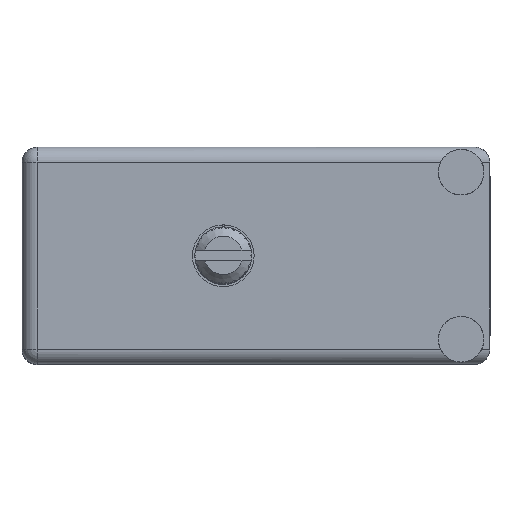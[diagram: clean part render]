
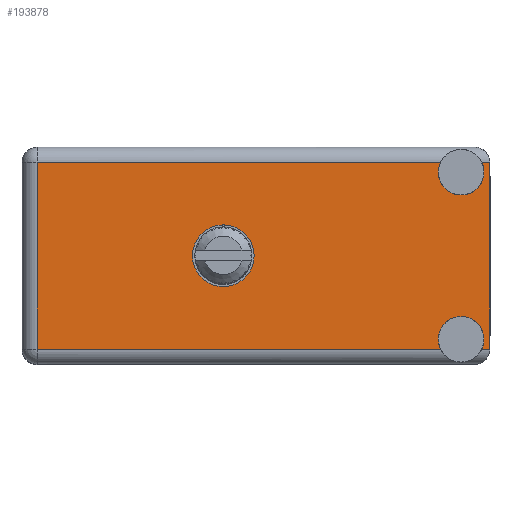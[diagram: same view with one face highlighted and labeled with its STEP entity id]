
A CAD part, top view. The second image highlights one B-rep face of the part: STEP entity #193878.
In plain terms, the highlighted face is planar.
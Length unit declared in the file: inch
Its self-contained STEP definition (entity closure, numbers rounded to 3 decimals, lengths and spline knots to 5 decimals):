
#703 = ORIENTED_EDGE ( 'NONE', *, *, #146968, .T. ) ;
#1648 = EDGE_CURVE ( 'NONE', #53307, #100496, #67177, .T. ) ;
#1703 = CIRCLE ( 'NONE', #99555, 0.1015 ) ;
#3553 = CARTESIAN_POINT ( 'NONE',  ( 0., 0.906, -0.665 ) ) ;
#8073 = DIRECTION ( 'NONE',  ( 0., 0., 1. ) ) ;
#11245 = CARTESIAN_POINT ( 'NONE',  ( 1.539, 0.906, -0.05 ) ) ;
#12957 = CARTESIAN_POINT ( 'NONE',  ( 0.6625, 0.906, -0.3575 ) ) ;
#14248 = CARTESIAN_POINT ( 'NONE',  ( 0.6625, 0.906, -0.459 ) ) ;
#14769 = ORIENTED_EDGE ( 'NONE', *, *, #183050, .F. ) ;
#20275 = VERTEX_POINT ( 'NONE', #14248 ) ;
#21609 = ORIENTED_EDGE ( 'NONE', *, *, #87381, .F. ) ;
#32112 = ORIENTED_EDGE ( 'NONE', *, *, #156382, .F. ) ;
#32458 = AXIS2_PLACEMENT_3D ( 'NONE', #95617, #155891, #96591 ) ;
#45005 = LINE ( 'NONE', #119097, #183199 ) ;
#48723 = CARTESIAN_POINT ( 'NONE',  ( 1.37741, 0.906, -0.05 ) ) ;
#49349 = CARTESIAN_POINT ( 'NONE',  ( 1.445, 0.906, -0.5575 ) ) ;
#52432 = CARTESIAN_POINT ( 'NONE',  ( 1.539, 0.906, -0.05 ) ) ;
#53307 = VERTEX_POINT ( 'NONE', #184322 ) ;
#53996 = DIRECTION ( 'NONE',  ( 0., 1., 0. ) ) ;
#55192 = CARTESIAN_POINT ( 'NONE',  ( 1.445, 0.906, -0.0825 ) ) ;
#55344 = VERTEX_POINT ( 'NONE', #49349 ) ;
#56175 = CIRCLE ( 'NONE', #191800, 0.075 ) ;
#57451 = DIRECTION ( 'NONE',  ( 0., 0., 1. ) ) ;
#59532 = EDGE_CURVE ( 'NONE', #158569, #181998, #45005, .T. ) ;
#60817 = VERTEX_POINT ( 'NONE', #178645 ) ;
#60821 = CIRCLE ( 'NONE', #108025, 0.1015 ) ;
#61886 = LINE ( 'NONE', #3553, #70765 ) ;
#63030 = VECTOR ( 'NONE', #103470, 39.37008 ) ;
#66276 = VERTEX_POINT ( 'NONE', #160468 ) ;
#66916 = FACE_BOUND ( 'NONE', #130423, .T. ) ;
#67177 = CIRCLE ( 'NONE', #32458, 0.075 ) ;
#67369 = CARTESIAN_POINT ( 'NONE',  ( 1.445, 0.906, -0.6325 ) ) ;
#67613 = ORIENTED_EDGE ( 'NONE', *, *, #1648, .F. ) ;
#68132 = EDGE_CURVE ( 'NONE', #60817, #158569, #134665, .T. ) ;
#70520 = VERTEX_POINT ( 'NONE', #84397 ) ;
#70765 = VECTOR ( 'NONE', #122090, 39.37008 ) ;
#71194 = CIRCLE ( 'NONE', #184795, 0.075 ) ;
#75678 = DIRECTION ( 'NONE',  ( 0., 0., 1. ) ) ;
#79089 = DIRECTION ( 'NONE',  ( -1., 0., 0. ) ) ;
#79803 = LINE ( 'NONE', #182551, #167916 ) ;
#84397 = CARTESIAN_POINT ( 'NONE',  ( 0.6625, 0.906, -0.256 ) ) ;
#85857 = DIRECTION ( 'NONE',  ( 0., 1., 0. ) ) ;
#87381 = EDGE_CURVE ( 'NONE', #176764, #139193, #79803, .T. ) ;
#95566 = DIRECTION ( 'NONE',  ( 0., 0., 1. ) ) ;
#95617 = CARTESIAN_POINT ( 'NONE',  ( 1.445, 0.906, -0.0825 ) ) ;
#96591 = DIRECTION ( 'NONE',  ( 0., 0., 1. ) ) ;
#96902 = VECTOR ( 'NONE', #79089, 39.37008 ) ;
#98404 = EDGE_CURVE ( 'NONE', #181998, #100496, #193363, .T. ) ;
#99501 = ORIENTED_EDGE ( 'NONE', *, *, #113482, .F. ) ;
#99555 = AXIS2_PLACEMENT_3D ( 'NONE', #169833, #166939, #108580 ) ;
#100496 = VERTEX_POINT ( 'NONE', #48723 ) ;
#103470 = DIRECTION ( 'NONE',  ( 1., 0., 0. ) ) ;
#108025 = AXIS2_PLACEMENT_3D ( 'NONE', #12957, #192759, #57451 ) ;
#108580 = DIRECTION ( 'NONE',  ( 0., 0., 1. ) ) ;
#113482 = EDGE_CURVE ( 'NONE', #60817, #55344, #56175, .T. ) ;
#114236 = DIRECTION ( 'NONE',  ( 0., 0., 1. ) ) ;
#115266 = DIRECTION ( 'NONE',  ( 0., 0., 1. ) ) ;
#115427 = DIRECTION ( 'NONE',  ( 0., 0., 1. ) ) ;
#118002 = ORIENTED_EDGE ( 'NONE', *, *, #135818, .T. ) ;
#118154 = ORIENTED_EDGE ( 'NONE', *, *, #59532, .T. ) ;
#119097 = CARTESIAN_POINT ( 'NONE',  ( 0.05, 0.906, -0.715 ) ) ;
#122090 = DIRECTION ( 'NONE',  ( -1., 0., 0. ) ) ;
#127576 = DIRECTION ( 'NONE',  ( 0., 1., 0. ) ) ;
#129082 = PLANE ( 'NONE',  #134290 ) ;
#130423 = EDGE_LOOP ( 'NONE', ( #32112, #137603 ) ) ;
#131162 = CARTESIAN_POINT ( 'NONE',  ( 1.539, 0.906, -0.05 ) ) ;
#134290 = AXIS2_PLACEMENT_3D ( 'NONE', #188364, #53996, #114236 ) ;
#134665 = LINE ( 'NONE', #194911, #96902 ) ;
#135818 = EDGE_CURVE ( 'NONE', #176764, #164476, #61886, .T. ) ;
#137603 = ORIENTED_EDGE ( 'NONE', *, *, #179980, .F. ) ;
#139193 = VERTEX_POINT ( 'NONE', #11245 ) ;
#142045 = CARTESIAN_POINT ( 'NONE',  ( 1.445, 0.906, -0.6325 ) ) ;
#142686 = CARTESIAN_POINT ( 'NONE',  ( 0.05, 0.906, -0.05 ) ) ;
#143849 = AXIS2_PLACEMENT_3D ( 'NONE', #142045, #187429, #115266 ) ;
#146923 = ORIENTED_EDGE ( 'NONE', *, *, #98404, .T. ) ;
#146968 = EDGE_CURVE ( 'NONE', #66276, #139193, #187749, .T. ) ;
#150491 = EDGE_CURVE ( 'NONE', #66276, #53307, #71194, .T. ) ;
#155891 = DIRECTION ( 'NONE',  ( 0., 1., 0. ) ) ;
#156382 = EDGE_CURVE ( 'NONE', #70520, #20275, #60821, .T. ) ;
#156669 = ORIENTED_EDGE ( 'NONE', *, *, #68132, .T. ) ;
#156825 = FACE_OUTER_BOUND ( 'NONE', #163430, .T. ) ;
#158569 = VERTEX_POINT ( 'NONE', #192371 ) ;
#160468 = CARTESIAN_POINT ( 'NONE',  ( 1.51259, 0.906, -0.05 ) ) ;
#163430 = EDGE_LOOP ( 'NONE', ( #146923, #67613, #188663, #703, #21609, #118002, #14769, #99501, #156669, #118154 ) ) ;
#163984 = CARTESIAN_POINT ( 'NONE',  ( 1.539, 0.906, -0.665 ) ) ;
#164476 = VERTEX_POINT ( 'NONE', #195472 ) ;
#166939 = DIRECTION ( 'NONE',  ( 0., 1., 0. ) ) ;
#167916 = VECTOR ( 'NONE', #95566, 39.37008 ) ;
#169833 = CARTESIAN_POINT ( 'NONE',  ( 0.6625, 0.906, -0.3575 ) ) ;
#172325 = CIRCLE ( 'NONE', #143849, 0.075 ) ;
#176764 = VERTEX_POINT ( 'NONE', #163984 ) ;
#178645 = CARTESIAN_POINT ( 'NONE',  ( 1.37741, 0.906, -0.665 ) ) ;
#179980 = EDGE_CURVE ( 'NONE', #20275, #70520, #1703, .T. ) ;
#181998 = VERTEX_POINT ( 'NONE', #142686 ) ;
#182551 = CARTESIAN_POINT ( 'NONE',  ( 1.539, 0.906, 0. ) ) ;
#183050 = EDGE_CURVE ( 'NONE', #55344, #164476, #172325, .T. ) ;
#183199 = VECTOR ( 'NONE', #75678, 39.37008 ) ;
#184322 = CARTESIAN_POINT ( 'NONE',  ( 1.445, 0.906, -0.1575 ) ) ;
#184795 = AXIS2_PLACEMENT_3D ( 'NONE', #55192, #85857, #115427 ) ;
#187429 = DIRECTION ( 'NONE',  ( 0., 1., 0. ) ) ;
#187749 = LINE ( 'NONE', #52432, #191271 ) ;
#188364 = CARTESIAN_POINT ( 'NONE',  ( 0., 0.906, -0.715 ) ) ;
#188663 = ORIENTED_EDGE ( 'NONE', *, *, #150491, .F. ) ;
#190668 = DIRECTION ( 'NONE',  ( 1., 0., 0. ) ) ;
#191271 = VECTOR ( 'NONE', #190668, 39.37008 ) ;
#191800 = AXIS2_PLACEMENT_3D ( 'NONE', #67369, #127576, #8073 ) ;
#192371 = CARTESIAN_POINT ( 'NONE',  ( 0.05, 0.906, -0.665 ) ) ;
#192759 = DIRECTION ( 'NONE',  ( 0., 1., 0. ) ) ;
#193363 = LINE ( 'NONE', #131162, #63030 ) ;
#193878 = ADVANCED_FACE ( 'NONE', ( #66916, #156825 ), #129082, .T. ) ;
#194911 = CARTESIAN_POINT ( 'NONE',  ( 0., 0.906, -0.665 ) ) ;
#195472 = CARTESIAN_POINT ( 'NONE',  ( 1.51259, 0.906, -0.665 ) ) ;
